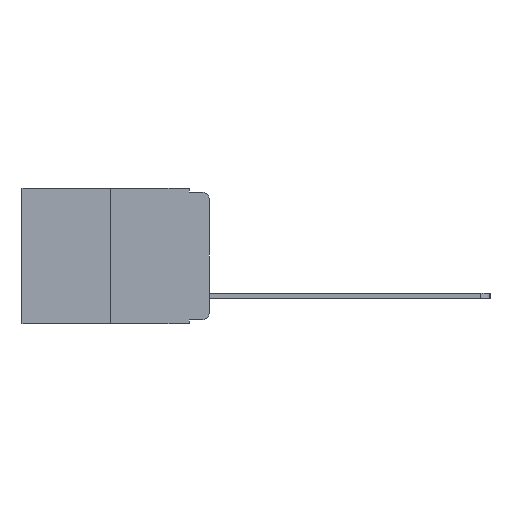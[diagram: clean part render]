
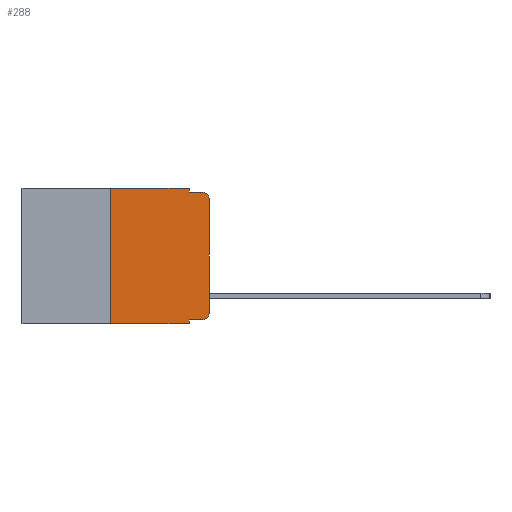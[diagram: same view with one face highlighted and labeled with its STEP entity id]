
A CAD part, left-side view. The second image highlights one B-rep face of the part: STEP entity #288.
In plain terms, the highlighted planar face has unit normal (-1, 0, 0).
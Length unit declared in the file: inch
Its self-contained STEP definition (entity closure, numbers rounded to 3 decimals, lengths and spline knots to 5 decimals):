
#58 = VECTOR ( 'NONE', #10595, 39.37008 ) ;
#210 = VECTOR ( 'NONE', #8803, 39.37008 ) ;
#234 = VERTEX_POINT ( 'NONE', #13097 ) ;
#288 = ADVANCED_FACE ( 'NONE', ( #7566 ), #9885, .F. ) ;
#956 = ORIENTED_EDGE ( 'NONE', *, *, #13292, .F. ) ;
#1359 = ORIENTED_EDGE ( 'NONE', *, *, #6205, .F. ) ;
#1467 = VERTEX_POINT ( 'NONE', #11435 ) ;
#1495 = CARTESIAN_POINT ( 'NONE',  ( 0., 0.051, -0.333 ) ) ;
#1864 = LINE ( 'NONE', #7173, #4925 ) ;
#2404 = VERTEX_POINT ( 'NONE', #8737 ) ;
#2537 = EDGE_CURVE ( 'NONE', #3683, #3903, #6284, .T. ) ;
#2798 = CIRCLE ( 'NONE', #5172, 0.02 ) ;
#3014 = DIRECTION ( 'NONE',  ( 0., -1., 0. ) ) ;
#3144 = DIRECTION ( 'NONE',  ( 0., 0., -1. ) ) ;
#3179 = CARTESIAN_POINT ( 'NONE',  ( 0., 0.051, -0.343 ) ) ;
#3284 = LINE ( 'NONE', #8577, #58 ) ;
#3648 = CARTESIAN_POINT ( 'NONE',  ( 0., 0.25, 0. ) ) ;
#3683 = VERTEX_POINT ( 'NONE', #9905 ) ;
#3903 = VERTEX_POINT ( 'NONE', #4173 ) ;
#4173 = CARTESIAN_POINT ( 'NONE',  ( 0., 0., -0.03 ) ) ;
#4484 = ORIENTED_EDGE ( 'NONE', *, *, #4942, .T. ) ;
#4921 = VERTEX_POINT ( 'NONE', #4976 ) ;
#4925 = VECTOR ( 'NONE', #8391, 39.37008 ) ;
#4942 = EDGE_CURVE ( 'NONE', #234, #13575, #12421, .T. ) ;
#4976 = CARTESIAN_POINT ( 'NONE',  ( 0., 0.02, -0.01 ) ) ;
#5172 = AXIS2_PLACEMENT_3D ( 'NONE', #9499, #10510, #10552 ) ;
#5523 = CARTESIAN_POINT ( 'NONE',  ( 0., 0., 0. ) ) ;
#5530 = EDGE_CURVE ( 'NONE', #3903, #4921, #2798, .T. ) ;
#5630 = DIRECTION ( 'NONE',  ( 0., 0., 1. ) ) ;
#5653 = CARTESIAN_POINT ( 'NONE',  ( 0., 0.051, -0.01 ) ) ;
#5723 = CARTESIAN_POINT ( 'NONE',  ( 0., 0.473, -0.343 ) ) ;
#5776 = EDGE_CURVE ( 'NONE', #8284, #12496, #1864, .T. ) ;
#5825 = DIRECTION ( 'NONE',  ( 0., 0., -1. ) ) ;
#6182 = CARTESIAN_POINT ( 'NONE',  ( 0., 0.02, -0.313 ) ) ;
#6205 = EDGE_CURVE ( 'NONE', #234, #2404, #12687, .T. ) ;
#6207 = DIRECTION ( 'NONE',  ( 1., 0., 0. ) ) ;
#6284 = LINE ( 'NONE', #5523, #210 ) ;
#6288 = CARTESIAN_POINT ( 'NONE',  ( 0., 0.051, -0.01 ) ) ;
#6933 = EDGE_CURVE ( 'NONE', #8284, #13575, #3284, .T. ) ;
#6943 = EDGE_LOOP ( 'NONE', ( #12754, #13370, #11405, #11715, #956, #1359, #4484, #7287, #7644, #7963 ) ) ;
#7045 = CARTESIAN_POINT ( 'NONE',  ( 0., 0.02, -0.333 ) ) ;
#7173 = CARTESIAN_POINT ( 'NONE',  ( 0., 0.051, -0.333 ) ) ;
#7287 = ORIENTED_EDGE ( 'NONE', *, *, #6933, .F. ) ;
#7566 = FACE_OUTER_BOUND ( 'NONE', #6943, .T. ) ;
#7644 = ORIENTED_EDGE ( 'NONE', *, *, #5776, .T. ) ;
#7689 = LINE ( 'NONE', #8936, #12658 ) ;
#7935 = EDGE_CURVE ( 'NONE', #12496, #3683, #11275, .T. ) ;
#7963 = ORIENTED_EDGE ( 'NONE', *, *, #7935, .T. ) ;
#8125 = VECTOR ( 'NONE', #3014, 39.37008 ) ;
#8284 = VERTEX_POINT ( 'NONE', #1495 ) ;
#8383 = EDGE_CURVE ( 'NONE', #1467, #10701, #7689, .T. ) ;
#8391 = DIRECTION ( 'NONE',  ( 0., -1., 0. ) ) ;
#8577 = CARTESIAN_POINT ( 'NONE',  ( 0., 0.051, 0. ) ) ;
#8629 = AXIS2_PLACEMENT_3D ( 'NONE', #6182, #9536, #3144 ) ;
#8737 = CARTESIAN_POINT ( 'NONE',  ( 0., 0.25, 0. ) ) ;
#8803 = DIRECTION ( 'NONE',  ( 0., 0., 1. ) ) ;
#8936 = CARTESIAN_POINT ( 'NONE',  ( 0., 0.051, 0. ) ) ;
#9499 = CARTESIAN_POINT ( 'NONE',  ( 0., 0.02, -0.03 ) ) ;
#9536 = DIRECTION ( 'NONE',  ( -1., 0., 0. ) ) ;
#9885 = PLANE ( 'NONE',  #11772 ) ;
#9905 = CARTESIAN_POINT ( 'NONE',  ( 0., 0., -0.313 ) ) ;
#10113 = VECTOR ( 'NONE', #5630, 39.37008 ) ;
#10272 = DIRECTION ( 'NONE',  ( 0., 0., -1. ) ) ;
#10406 = EDGE_CURVE ( 'NONE', #10701, #4921, #13376, .T. ) ;
#10510 = DIRECTION ( 'NONE',  ( -1., 0., 0. ) ) ;
#10552 = DIRECTION ( 'NONE',  ( 0., 0., -1. ) ) ;
#10595 = DIRECTION ( 'NONE',  ( 0., 0., -1. ) ) ;
#10701 = VERTEX_POINT ( 'NONE', #5653 ) ;
#10732 = DIRECTION ( 'NONE',  ( 0., -1., 0. ) ) ;
#11225 = VECTOR ( 'NONE', #13068, 39.37008 ) ;
#11275 = CIRCLE ( 'NONE', #8629, 0.02 ) ;
#11405 = ORIENTED_EDGE ( 'NONE', *, *, #10406, .F. ) ;
#11435 = CARTESIAN_POINT ( 'NONE',  ( 0., 0.051, 0. ) ) ;
#11715 = ORIENTED_EDGE ( 'NONE', *, *, #8383, .F. ) ;
#11772 = AXIS2_PLACEMENT_3D ( 'NONE', #13647, #6207, #10272 ) ;
#12101 = CARTESIAN_POINT ( 'NONE',  ( 0., 0.473, 0. ) ) ;
#12421 = LINE ( 'NONE', #5723, #12720 ) ;
#12496 = VERTEX_POINT ( 'NONE', #7045 ) ;
#12658 = VECTOR ( 'NONE', #5825, 39.37008 ) ;
#12687 = LINE ( 'NONE', #3648, #10113 ) ;
#12720 = VECTOR ( 'NONE', #10732, 39.37008 ) ;
#12754 = ORIENTED_EDGE ( 'NONE', *, *, #2537, .T. ) ;
#13068 = DIRECTION ( 'NONE',  ( 0., -1., 0. ) ) ;
#13097 = CARTESIAN_POINT ( 'NONE',  ( 0., 0.25, -0.343 ) ) ;
#13292 = EDGE_CURVE ( 'NONE', #2404, #1467, #13786, .T. ) ;
#13370 = ORIENTED_EDGE ( 'NONE', *, *, #5530, .T. ) ;
#13376 = LINE ( 'NONE', #6288, #8125 ) ;
#13575 = VERTEX_POINT ( 'NONE', #3179 ) ;
#13647 = CARTESIAN_POINT ( 'NONE',  ( 0., 0.473, 0. ) ) ;
#13786 = LINE ( 'NONE', #12101, #11225 ) ;
